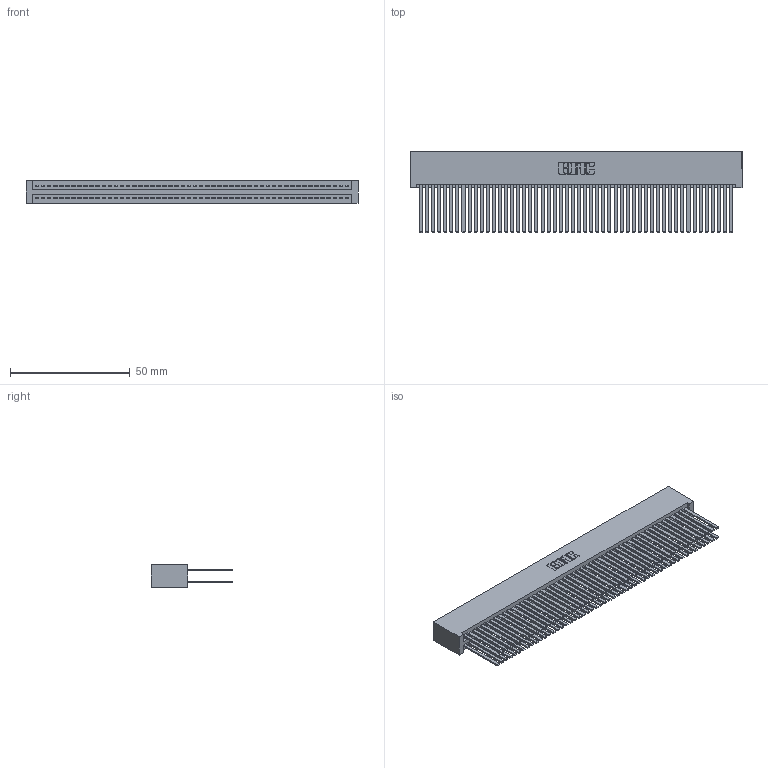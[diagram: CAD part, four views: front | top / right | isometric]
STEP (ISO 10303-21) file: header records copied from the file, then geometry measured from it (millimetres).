
FILE_DESCRIPTION (( 'STEP AP203' ), '1' );
FILE_NAME ('395-104-544-201.STEP', '2018-11-30T13:34:34', ( '' ), ( '' ), 'SwSTEP 2.0', 'SolidWorks 2016', '' );
FILE_SCHEMA (( 'CONFIG_CONTROL_DESIGN' ));
Length unit declared in the file: inch
Products named in the file (3): 345-292-001_345-293-144; 345 Part_No Mounting Lugs; 395-104-544-201
Assembly tree (105 placements, depth 2):
  395-104-544-201
    345 Part_No Mounting Lugs
    345-292-001_345-293-144  x104
Bounding box: 138.68 x 33.96 x 9.4 mm (x, y, z)
Volume: 15638.5 mm3; surface area: 27886.3 mm2
Topology: 105 solids, 105 shells, 4694 faces, 13941 edges, 9154 vertices
Faces by surface type: plane 3092, cylinder 1602
Entity records: 38993 total; most frequent: CARTESIAN_POINT 6524, ORIENTED_EDGE 6458, DIRECTION 5733, EDGE_CURVE 3229, LINE 2901, VECTOR 2901, VERTEX_POINT 2150, AXIS2_PLACEMENT_3D 1416
